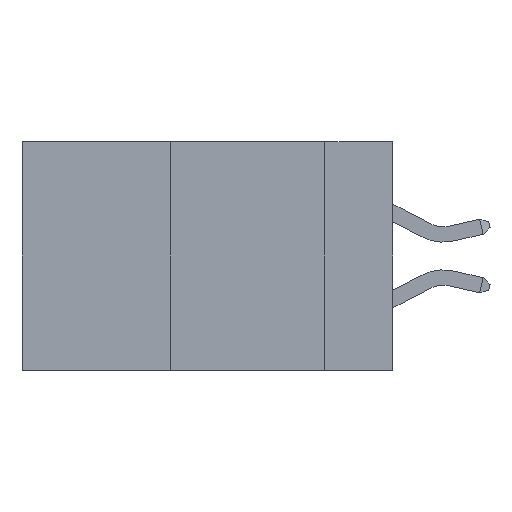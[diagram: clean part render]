
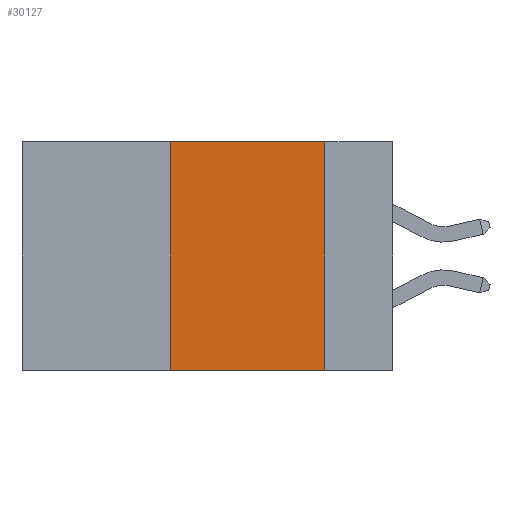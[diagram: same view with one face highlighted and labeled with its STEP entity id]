
A CAD part, left-side view. The second image highlights one B-rep face of the part: STEP entity #30127.
In plain terms, the highlighted planar face has unit normal (-1, 0, 0).
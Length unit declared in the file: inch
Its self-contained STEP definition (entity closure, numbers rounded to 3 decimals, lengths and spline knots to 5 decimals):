
#24 = CARTESIAN_POINT ( 'NONE',  ( 0., 0.36, 0. ) ) ;
#1146 = ORIENTED_EDGE ( 'NONE', *, *, #19507, .T. ) ;
#2221 = LINE ( 'NONE', #24, #25560 ) ;
#2903 = DIRECTION ( 'NONE',  ( 0., 0., -1. ) ) ;
#4489 = VECTOR ( 'NONE', #2903, 39.37008 ) ;
#4553 = CARTESIAN_POINT ( 'NONE',  ( 0., 0.11, -0.37 ) ) ;
#5235 = ORIENTED_EDGE ( 'NONE', *, *, #17229, .F. ) ;
#6200 = DIRECTION ( 'NONE',  ( 0., -1., 0. ) ) ;
#6627 = VECTOR ( 'NONE', #6200, 39.37008 ) ;
#7144 = LINE ( 'NONE', #19933, #20512 ) ;
#7989 = CARTESIAN_POINT ( 'NONE',  ( 0., 0.11, 0. ) ) ;
#8669 = LINE ( 'NONE', #10856, #4489 ) ;
#10618 = DIRECTION ( 'NONE',  ( 0., 0., -1. ) ) ;
#10622 = AXIS2_PLACEMENT_3D ( 'NONE', #26691, #10967, #10618 ) ;
#10856 = CARTESIAN_POINT ( 'NONE',  ( 0., 0.11, 0. ) ) ;
#10967 = DIRECTION ( 'NONE',  ( 1., 0., 0. ) ) ;
#12519 = CARTESIAN_POINT ( 'NONE',  ( 0., 0.36, -0.37 ) ) ;
#12894 = CARTESIAN_POINT ( 'NONE',  ( 0., 0.36, 0. ) ) ;
#17229 = EDGE_CURVE ( 'NONE', #33799, #31299, #2221, .T. ) ;
#17354 = DIRECTION ( 'NONE',  ( 0., -1., 0. ) ) ;
#18322 = EDGE_CURVE ( 'NONE', #31299, #28913, #7144, .T. ) ;
#18724 = DIRECTION ( 'NONE',  ( 0., 0., 1. ) ) ;
#19507 = EDGE_CURVE ( 'NONE', #33799, #25615, #33813, .T. ) ;
#19933 = CARTESIAN_POINT ( 'NONE',  ( 0., 0.6, 0. ) ) ;
#20512 = VECTOR ( 'NONE', #17354, 39.37008 ) ;
#24037 = PLANE ( 'NONE',  #10622 ) ;
#25560 = VECTOR ( 'NONE', #18724, 39.37008 ) ;
#25615 = VERTEX_POINT ( 'NONE', #4553 ) ;
#26691 = CARTESIAN_POINT ( 'NONE',  ( 0., 0.6, 0. ) ) ;
#28913 = VERTEX_POINT ( 'NONE', #7989 ) ;
#30117 = EDGE_CURVE ( 'NONE', #28913, #25615, #8669, .T. ) ;
#30127 = ADVANCED_FACE ( 'NONE', ( #32084 ), #24037, .F. ) ;
#31299 = VERTEX_POINT ( 'NONE', #12894 ) ;
#32084 = FACE_OUTER_BOUND ( 'NONE', #33909, .T. ) ;
#32734 = CARTESIAN_POINT ( 'NONE',  ( 0., 0.6, -0.37 ) ) ;
#33799 = VERTEX_POINT ( 'NONE', #12519 ) ;
#33813 = LINE ( 'NONE', #32734, #6627 ) ;
#33870 = ORIENTED_EDGE ( 'NONE', *, *, #30117, .F. ) ;
#33909 = EDGE_LOOP ( 'NONE', ( #33870, #34590, #5235, #1146 ) ) ;
#34590 = ORIENTED_EDGE ( 'NONE', *, *, #18322, .F. ) ;
